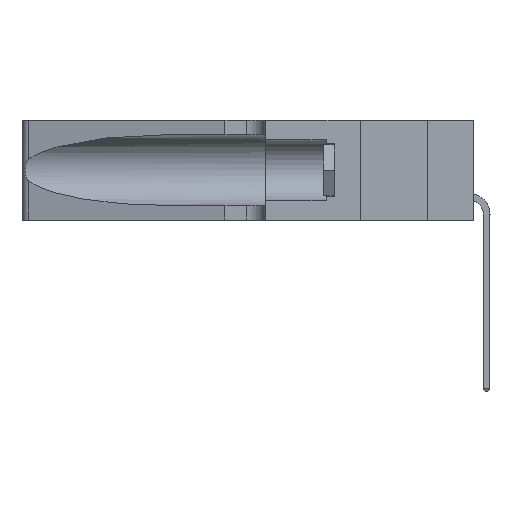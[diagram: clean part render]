
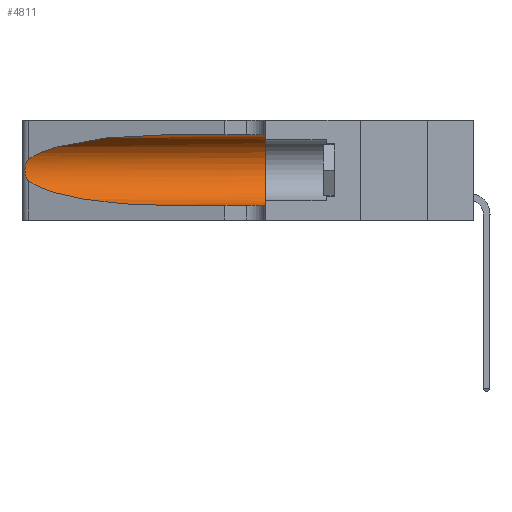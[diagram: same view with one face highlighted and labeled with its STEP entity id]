
A CAD part, left-side view. The second image highlights one B-rep face of the part: STEP entity #4811.
In plain terms, the highlighted cylindrical face has radius 3.308 mm (diameter 6.617 mm), a partial arc.
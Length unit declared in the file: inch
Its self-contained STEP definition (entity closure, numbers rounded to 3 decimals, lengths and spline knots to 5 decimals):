
#653 = DIRECTION ( 'NONE',  ( 0., -1., 0. ) ) ;
#791 = CYLINDRICAL_SURFACE ( 'NONE', #5477, 0.13025 ) ;
#882 = DIRECTION ( 'NONE',  ( 0., -1., 0. ) ) ;
#949 = CARTESIAN_POINT ( 'NONE',  ( 0.25487, 1.22718, 0.22369 ) ) ;
#1327 = CARTESIAN_POINT ( 'NONE',  ( 0.26075, 1.23896, 0.19203 ) ) ;
#1605 = VERTEX_POINT ( 'NONE', #18430 ) ;
#2153 = ORIENTED_EDGE ( 'NONE', *, *, #6746, .F. ) ;
#2642 = EDGE_CURVE ( 'NONE', #14136, #4048, #5493, .T. ) ;
#3756 = VECTOR ( 'NONE', #882, 39.37008 ) ;
#3882 = CARTESIAN_POINT ( 'NONE',  ( 0.1305, 1.61858, 0.31525 ) ) ;
#4013 = EDGE_LOOP ( 'NONE', ( #17372, #4395, #19648, #18581, #19145, #2153 ) ) ;
#4048 = VERTEX_POINT ( 'NONE', #949 ) ;
#4364 = EDGE_CURVE ( 'NONE', #10153, #1605, #11999, .T. ) ;
#4395 = ORIENTED_EDGE ( 'NONE', *, *, #14025, .T. ) ;
#4559 = CARTESIAN_POINT ( 'NONE',  ( 0.18966, 0.96281, 0.31525 ) ) ;
#4811 = ADVANCED_FACE ( 'NONE', ( #6268 ), #791, .F. ) ;
#5477 = AXIS2_PLACEMENT_3D ( 'NONE', #11583, #11520, #9859 ) ;
#5493 =( BOUNDED_CURVE ( )  B_SPLINE_CURVE ( 3, ( #12022, #4559, #16759, #12232 ),
 .UNSPECIFIED., .F., .F. ) 
 B_SPLINE_CURVE_WITH_KNOTS ( ( 4, 4 ),
 ( 1.5708, 2.84003 ),
 .UNSPECIFIED. ) 
 CURVE ( )  GEOMETRIC_REPRESENTATION_ITEM ( )  RATIONAL_B_SPLINE_CURVE ( ( 1., 0.87, 0.87, 1. ) ) 
 REPRESENTATION_ITEM ( '' )  );
#5603 = CARTESIAN_POINT ( 'NONE',  ( 0.1305, 0.72297, 0.05475 ) ) ;
#5815 = CARTESIAN_POINT ( 'NONE',  ( 0.18966, 0.96281, 0.05475 ) ) ;
#5874 = CARTESIAN_POINT ( 'NONE',  ( 0.1305, 0.72297, 0.05475 ) ) ;
#5904 = CARTESIAN_POINT ( 'NONE',  ( 0.25787, 1.23484, 0.2124 ) ) ;
#6041 = CARTESIAN_POINT ( 'NONE',  ( 0.25639, 1.23184, 0.21858 ) ) ;
#6268 = FACE_OUTER_BOUND ( 'NONE', #4013, .T. ) ;
#6348 = B_SPLINE_CURVE_WITH_KNOTS ( 'NONE', 3,
 ( #7593, #18182, #6041, #5904, #9120, #8510, #1327, #7533, #18117, #12114, #11917, #18042, #12041, #9052 ),
 .UNSPECIFIED., .F., .F.,
 ( 4, 2, 2, 2, 2, 2, 4 ),
 ( 0., 0.00027, 0.00053, 0.00107, 0.0016, 0.00187, 0.00214 ),
 .UNSPECIFIED. ) ;
#6746 = EDGE_CURVE ( 'NONE', #14136, #15786, #15414, .T. ) ;
#7533 = CARTESIAN_POINT ( 'NONE',  ( 0.26075, 1.23896, 0.178 ) ) ;
#7593 = CARTESIAN_POINT ( 'NONE',  ( 0.25487, 1.22718, 0.22369 ) ) ;
#8510 = CARTESIAN_POINT ( 'NONE',  ( 0.26018, 1.23835, 0.19895 ) ) ;
#9052 = CARTESIAN_POINT ( 'NONE',  ( 0.25487, 1.22718, 0.14631 ) ) ;
#9120 = CARTESIAN_POINT ( 'NONE',  ( 0.25854, 1.2359, 0.20912 ) ) ;
#9859 = DIRECTION ( 'NONE',  ( 0., 0., -1. ) ) ;
#10153 = VERTEX_POINT ( 'NONE', #5603 ) ;
#10352 = CARTESIAN_POINT ( 'NONE',  ( 0.2373, 1.15595, 0.08982 ) ) ;
#10742 =( BOUNDED_CURVE ( )  B_SPLINE_CURVE ( 3, ( #15011, #10352, #5815, #5874 ),
 .UNSPECIFIED., .F., .T. ) 
 B_SPLINE_CURVE_WITH_KNOTS ( ( 4, 4 ),
 ( 3.44316, 4.71239 ),
 .UNSPECIFIED. ) 
 CURVE ( )  GEOMETRIC_REPRESENTATION_ITEM ( )  RATIONAL_B_SPLINE_CURVE ( ( 1., 0.87, 0.87, 1. ) ) 
 REPRESENTATION_ITEM ( '' )  );
#11101 = AXIS2_PLACEMENT_3D ( 'NONE', #11561, #17800, #19359 ) ;
#11520 = DIRECTION ( 'NONE',  ( 0., -1., 0. ) ) ;
#11561 = CARTESIAN_POINT ( 'NONE',  ( 0.1305, 0.35, 0.185 ) ) ;
#11583 = CARTESIAN_POINT ( 'NONE',  ( 0.1305, 1.61858, 0.185 ) ) ;
#11917 = CARTESIAN_POINT ( 'NONE',  ( 0.25789, 1.23486, 0.15765 ) ) ;
#11924 = VERTEX_POINT ( 'NONE', #17935 ) ;
#11999 = LINE ( 'NONE', #15904, #13445 ) ;
#12022 = CARTESIAN_POINT ( 'NONE',  ( 0.1305, 0.72297, 0.31525 ) ) ;
#12041 = CARTESIAN_POINT ( 'NONE',  ( 0.25555, 1.22993, 0.14849 ) ) ;
#12114 = CARTESIAN_POINT ( 'NONE',  ( 0.25856, 1.23593, 0.16098 ) ) ;
#12232 = CARTESIAN_POINT ( 'NONE',  ( 0.25487, 1.22718, 0.22369 ) ) ;
#12319 = CARTESIAN_POINT ( 'NONE',  ( 0.1305, 0.72297, 0.31525 ) ) ;
#13218 = CIRCLE ( 'NONE', #11101, 0.13025 ) ;
#13271 = EDGE_CURVE ( 'NONE', #15786, #1605, #13218, .T. ) ;
#13445 = VECTOR ( 'NONE', #653, 39.37008 ) ;
#14025 = EDGE_CURVE ( 'NONE', #4048, #11924, #6348, .T. ) ;
#14136 = VERTEX_POINT ( 'NONE', #12319 ) ;
#15011 = CARTESIAN_POINT ( 'NONE',  ( 0.25487, 1.22718, 0.14631 ) ) ;
#15414 = LINE ( 'NONE', #3882, #3756 ) ;
#15680 = EDGE_CURVE ( 'NONE', #11924, #10153, #10742, .T. ) ;
#15786 = VERTEX_POINT ( 'NONE', #18278 ) ;
#15904 = CARTESIAN_POINT ( 'NONE',  ( 0.1305, 1.61858, 0.05475 ) ) ;
#16759 = CARTESIAN_POINT ( 'NONE',  ( 0.2373, 1.15595, 0.28018 ) ) ;
#17372 = ORIENTED_EDGE ( 'NONE', *, *, #2642, .T. ) ;
#17800 = DIRECTION ( 'NONE',  ( 0., 1., 0. ) ) ;
#17935 = CARTESIAN_POINT ( 'NONE',  ( 0.25487, 1.22718, 0.14631 ) ) ;
#18042 = CARTESIAN_POINT ( 'NONE',  ( 0.25639, 1.23186, 0.15144 ) ) ;
#18117 = CARTESIAN_POINT ( 'NONE',  ( 0.26017, 1.23833, 0.17102 ) ) ;
#18182 = CARTESIAN_POINT ( 'NONE',  ( 0.25555, 1.22994, 0.2215 ) ) ;
#18278 = CARTESIAN_POINT ( 'NONE',  ( 0.1305, 0.35, 0.31525 ) ) ;
#18430 = CARTESIAN_POINT ( 'NONE',  ( 0.1305, 0.35, 0.05475 ) ) ;
#18581 = ORIENTED_EDGE ( 'NONE', *, *, #4364, .T. ) ;
#19145 = ORIENTED_EDGE ( 'NONE', *, *, #13271, .F. ) ;
#19359 = DIRECTION ( 'NONE',  ( 0., 0., 1. ) ) ;
#19648 = ORIENTED_EDGE ( 'NONE', *, *, #15680, .T. ) ;
